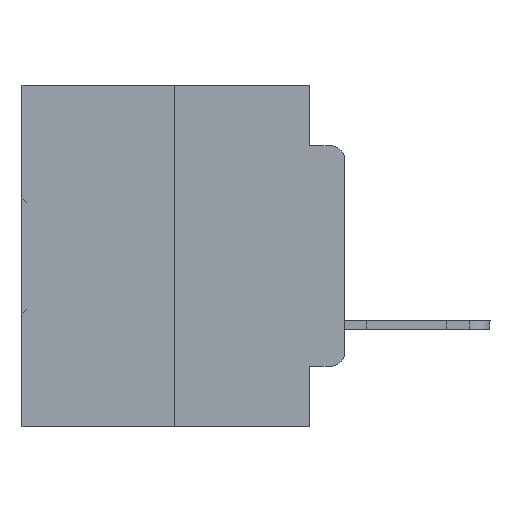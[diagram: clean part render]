
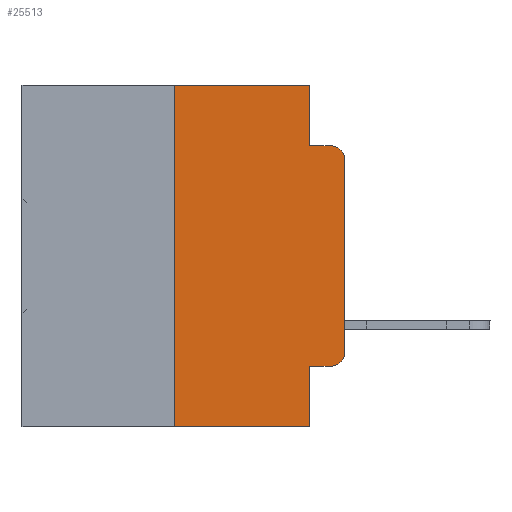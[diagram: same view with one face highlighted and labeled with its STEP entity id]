
A CAD part, left-side view. The second image highlights one B-rep face of the part: STEP entity #25513.
In plain terms, the highlighted planar face has unit normal (-1, 0, 0).
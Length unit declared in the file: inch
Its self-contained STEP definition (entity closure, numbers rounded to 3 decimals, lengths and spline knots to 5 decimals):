
#707 = CARTESIAN_POINT ( 'NONE',  ( 0., 0.051, 0. ) ) ;
#814 = VERTEX_POINT ( 'NONE', #12489 ) ;
#961 = ORIENTED_EDGE ( 'NONE', *, *, #29975, .F. ) ;
#980 = FACE_OUTER_BOUND ( 'NONE', #25738, .T. ) ;
#1062 = CARTESIAN_POINT ( 'NONE',  ( 0., 0., 0. ) ) ;
#1128 = LINE ( 'NONE', #1062, #28394 ) ;
#1820 = LINE ( 'NONE', #707, #14706 ) ;
#1832 = CIRCLE ( 'NONE', #11081, 0.02 ) ;
#2325 = CARTESIAN_POINT ( 'NONE',  ( 0., 0.02, -0.3915 ) ) ;
#2470 = VECTOR ( 'NONE', #23913, 39.37008 ) ;
#2676 = ORIENTED_EDGE ( 'NONE', *, *, #4083, .T. ) ;
#3942 = VERTEX_POINT ( 'NONE', #10549 ) ;
#4083 = EDGE_CURVE ( 'NONE', #13069, #12942, #16957, .T. ) ;
#4904 = CARTESIAN_POINT ( 'NONE',  ( 0., 0.473, 0. ) ) ;
#5049 = EDGE_CURVE ( 'NONE', #13069, #21639, #16435, .T. ) ;
#5063 = VECTOR ( 'NONE', #9331, 39.37008 ) ;
#5117 = VERTEX_POINT ( 'NONE', #13021 ) ;
#6530 = CARTESIAN_POINT ( 'NONE',  ( 0., 0.25, -0.5 ) ) ;
#6702 = VERTEX_POINT ( 'NONE', #6530 ) ;
#7152 = DIRECTION ( 'NONE',  ( 0., 0., -1. ) ) ;
#7389 = DIRECTION ( 'NONE',  ( 0., 0., -1. ) ) ;
#7689 = ORIENTED_EDGE ( 'NONE', *, *, #16724, .F. ) ;
#7852 = CARTESIAN_POINT ( 'NONE',  ( 0., 0.25, 0. ) ) ;
#8220 = VERTEX_POINT ( 'NONE', #7852 ) ;
#9118 = CARTESIAN_POINT ( 'NONE',  ( 0., 0.02, -0.4115 ) ) ;
#9331 = DIRECTION ( 'NONE',  ( 0., 0., 1. ) ) ;
#10128 = DIRECTION ( 'NONE',  ( 0., 0., -1. ) ) ;
#10549 = CARTESIAN_POINT ( 'NONE',  ( 0., 0.02, -0.0885 ) ) ;
#10865 = VECTOR ( 'NONE', #32374, 39.37008 ) ;
#11081 = AXIS2_PLACEMENT_3D ( 'NONE', #22457, #12535, #7152 ) ;
#12378 = AXIS2_PLACEMENT_3D ( 'NONE', #2325, #30675, #10128 ) ;
#12489 = CARTESIAN_POINT ( 'NONE',  ( 0., 0.051, 0. ) ) ;
#12535 = DIRECTION ( 'NONE',  ( -1., 0., 0. ) ) ;
#12708 = DIRECTION ( 'NONE',  ( 0., 0., -1. ) ) ;
#12940 = ORIENTED_EDGE ( 'NONE', *, *, #21201, .T. ) ;
#12942 = VERTEX_POINT ( 'NONE', #9118 ) ;
#13021 = CARTESIAN_POINT ( 'NONE',  ( 0., 0., -0.1085 ) ) ;
#13053 = ORIENTED_EDGE ( 'NONE', *, *, #5049, .F. ) ;
#13069 = VERTEX_POINT ( 'NONE', #21554 ) ;
#13175 = VERTEX_POINT ( 'NONE', #16188 ) ;
#13278 = LINE ( 'NONE', #17095, #10865 ) ;
#14706 = VECTOR ( 'NONE', #29309, 39.37008 ) ;
#16188 = CARTESIAN_POINT ( 'NONE',  ( 0., 0.051, -0.0885 ) ) ;
#16306 = CARTESIAN_POINT ( 'NONE',  ( 0., 0.051, -0.5 ) ) ;
#16435 = LINE ( 'NONE', #22831, #19674 ) ;
#16458 = EDGE_CURVE ( 'NONE', #32885, #5117, #1128, .T. ) ;
#16724 = EDGE_CURVE ( 'NONE', #13175, #3942, #31933, .T. ) ;
#16919 = VECTOR ( 'NONE', #30029, 39.37008 ) ;
#16957 = LINE ( 'NONE', #28548, #2470 ) ;
#17048 = CARTESIAN_POINT ( 'NONE',  ( 0., 0.25, 0. ) ) ;
#17095 = CARTESIAN_POINT ( 'NONE',  ( 0., 0.473, 0. ) ) ;
#18050 = DIRECTION ( 'NONE',  ( 0., -1., 0. ) ) ;
#18478 = EDGE_CURVE ( 'NONE', #5117, #3942, #1832, .T. ) ;
#19403 = CIRCLE ( 'NONE', #12378, 0.02 ) ;
#19438 = EDGE_CURVE ( 'NONE', #12942, #32885, #19403, .T. ) ;
#19674 = VECTOR ( 'NONE', #12708, 39.37008 ) ;
#20139 = DIRECTION ( 'NONE',  ( 1., 0., 0. ) ) ;
#21201 = EDGE_CURVE ( 'NONE', #6702, #21639, #29723, .T. ) ;
#21554 = CARTESIAN_POINT ( 'NONE',  ( 0., 0.051, -0.4115 ) ) ;
#21639 = VERTEX_POINT ( 'NONE', #16306 ) ;
#22405 = CARTESIAN_POINT ( 'NONE',  ( 0., 0.473, -0.5 ) ) ;
#22457 = CARTESIAN_POINT ( 'NONE',  ( 0., 0.02, -0.1085 ) ) ;
#22831 = CARTESIAN_POINT ( 'NONE',  ( 0., 0.051, 0. ) ) ;
#23053 = LINE ( 'NONE', #17048, #5063 ) ;
#23913 = DIRECTION ( 'NONE',  ( 0., -1., 0. ) ) ;
#23991 = DIRECTION ( 'NONE',  ( 0., 0., 1. ) ) ;
#24121 = EDGE_CURVE ( 'NONE', #814, #13175, #1820, .T. ) ;
#24902 = ORIENTED_EDGE ( 'NONE', *, *, #18478, .T. ) ;
#25513 = ADVANCED_FACE ( 'NONE', ( #980 ), #27878, .F. ) ;
#25572 = ORIENTED_EDGE ( 'NONE', *, *, #24121, .F. ) ;
#25738 = EDGE_LOOP ( 'NONE', ( #27881, #24902, #7689, #25572, #28111, #961, #12940, #13053, #2676, #31962 ) ) ;
#27878 = PLANE ( 'NONE',  #31058 ) ;
#27881 = ORIENTED_EDGE ( 'NONE', *, *, #16458, .T. ) ;
#28023 = CARTESIAN_POINT ( 'NONE',  ( 0., 0.051, -0.0885 ) ) ;
#28111 = ORIENTED_EDGE ( 'NONE', *, *, #33024, .F. ) ;
#28394 = VECTOR ( 'NONE', #23991, 39.37008 ) ;
#28548 = CARTESIAN_POINT ( 'NONE',  ( 0., 0.051, -0.4115 ) ) ;
#29309 = DIRECTION ( 'NONE',  ( 0., 0., -1. ) ) ;
#29613 = CARTESIAN_POINT ( 'NONE',  ( 0., 0., -0.3915 ) ) ;
#29723 = LINE ( 'NONE', #22405, #16919 ) ;
#29975 = EDGE_CURVE ( 'NONE', #6702, #8220, #23053, .T. ) ;
#30029 = DIRECTION ( 'NONE',  ( 0., -1., 0. ) ) ;
#30675 = DIRECTION ( 'NONE',  ( -1., 0., 0. ) ) ;
#31058 = AXIS2_PLACEMENT_3D ( 'NONE', #4904, #20139, #7389 ) ;
#31933 = LINE ( 'NONE', #28023, #32338 ) ;
#31962 = ORIENTED_EDGE ( 'NONE', *, *, #19438, .T. ) ;
#32338 = VECTOR ( 'NONE', #18050, 39.37008 ) ;
#32374 = DIRECTION ( 'NONE',  ( 0., -1., 0. ) ) ;
#32885 = VERTEX_POINT ( 'NONE', #29613 ) ;
#33024 = EDGE_CURVE ( 'NONE', #8220, #814, #13278, .T. ) ;
